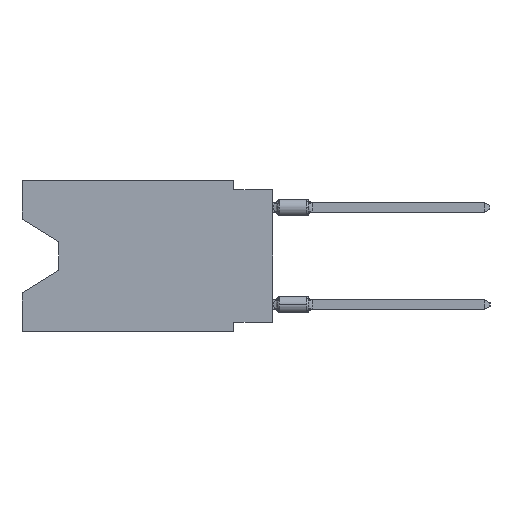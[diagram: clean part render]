
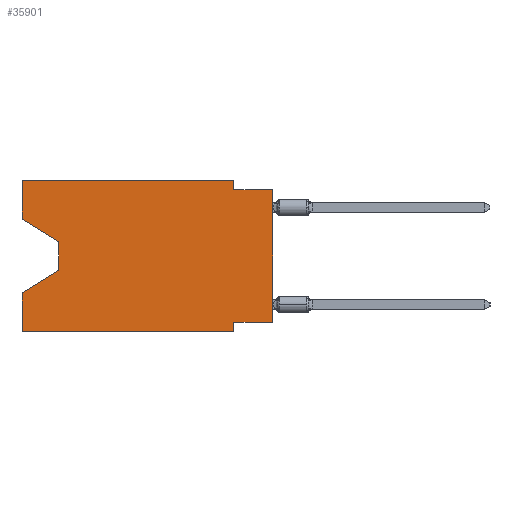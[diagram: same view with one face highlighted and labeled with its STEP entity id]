
A CAD part, left-side view. The second image highlights one B-rep face of the part: STEP entity #35901.
In plain terms, the highlighted planar face has unit normal (-1, 0, 0).
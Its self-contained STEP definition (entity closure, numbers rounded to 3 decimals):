
#434 = CARTESIAN_POINT ( 'NONE',  ( 0., 2.54, -9.271 ) ) ;
#891 = CARTESIAN_POINT ( 'NONE',  ( 0., 16.383, -9.906 ) ) ;
#1484 = LINE ( 'NONE', #5335, #4789 ) ;
#1598 = VECTOR ( 'NONE', #32664, 1000. ) ;
#1638 = CARTESIAN_POINT ( 'NONE',  ( 0., 2.54, -0.635 ) ) ;
#1687 = VERTEX_POINT ( 'NONE', #32587 ) ;
#2540 = VERTEX_POINT ( 'NONE', #35864 ) ;
#3015 = CARTESIAN_POINT ( 'NONE',  ( 0., 16.383, 0. ) ) ;
#3181 = DIRECTION ( 'NONE',  ( 0., -1., 0. ) ) ;
#3291 = DIRECTION ( 'NONE',  ( 0., 0., 1. ) ) ;
#3505 = CARTESIAN_POINT ( 'NONE',  ( 0., 16.383, 0. ) ) ;
#4196 = VERTEX_POINT ( 'NONE', #13522 ) ;
#4789 = VECTOR ( 'NONE', #21442, 1000. ) ;
#5096 = VECTOR ( 'NONE', #3291, 1000. ) ;
#5335 = CARTESIAN_POINT ( 'NONE',  ( 0., 0., 0. ) ) ;
#5982 = DIRECTION ( 'NONE',  ( 0., -1., 0. ) ) ;
#6082 = CARTESIAN_POINT ( 'NONE',  ( 0., 2.54, -9.906 ) ) ;
#6250 = LINE ( 'NONE', #3015, #32793 ) ;
#6885 = DIRECTION ( 'NONE',  ( 0., 0.855, -0.519 ) ) ;
#8403 = EDGE_CURVE ( 'NONE', #33445, #1687, #29652, .T. ) ;
#8707 = ORIENTED_EDGE ( 'NONE', *, *, #40645, .F. ) ;
#9124 = EDGE_CURVE ( 'NONE', #30574, #18743, #27374, .T. ) ;
#9193 = CARTESIAN_POINT ( 'NONE',  ( 0., 0., -0.635 ) ) ;
#9357 = EDGE_CURVE ( 'NONE', #30794, #33891, #23034, .T. ) ;
#9848 = CARTESIAN_POINT ( 'NONE',  ( 0., 0., -9.271 ) ) ;
#10131 = ORIENTED_EDGE ( 'NONE', *, *, #9357, .F. ) ;
#10392 = CARTESIAN_POINT ( 'NONE',  ( 0., 13.97, -4.013 ) ) ;
#10699 = AXIS2_PLACEMENT_3D ( 'NONE', #3505, #36114, #16602 ) ;
#10720 = VECTOR ( 'NONE', #6885, 1000. ) ;
#10819 = CARTESIAN_POINT ( 'NONE',  ( 0., 2.54, 0. ) ) ;
#11073 = CARTESIAN_POINT ( 'NONE',  ( 0., 16.383, 0. ) ) ;
#11210 = ORIENTED_EDGE ( 'NONE', *, *, #15955, .F. ) ;
#11588 = VERTEX_POINT ( 'NONE', #9848 ) ;
#12098 = LINE ( 'NONE', #35879, #12775 ) ;
#12408 = LINE ( 'NONE', #22470, #14924 ) ;
#12775 = VECTOR ( 'NONE', #42122, 1000. ) ;
#12973 = FACE_OUTER_BOUND ( 'NONE', #33775, .T. ) ;
#13182 = CARTESIAN_POINT ( 'NONE',  ( 0., 16.383, 0. ) ) ;
#13522 = CARTESIAN_POINT ( 'NONE',  ( 0., 0., -0.635 ) ) ;
#14281 = CARTESIAN_POINT ( 'NONE',  ( 0., 16.383, -2.546 ) ) ;
#14666 = VECTOR ( 'NONE', #3181, 1000. ) ;
#14673 = VECTOR ( 'NONE', #42078, 1000. ) ;
#14924 = VECTOR ( 'NONE', #35763, 1000. ) ;
#15955 = EDGE_CURVE ( 'NONE', #11588, #33445, #12408, .T. ) ;
#16110 = DIRECTION ( 'NONE',  ( 0., 0., 1. ) ) ;
#16602 = DIRECTION ( 'NONE',  ( 0., 0., -1. ) ) ;
#18743 = VERTEX_POINT ( 'NONE', #10819 ) ;
#19368 = VERTEX_POINT ( 'NONE', #22126 ) ;
#19757 = CARTESIAN_POINT ( 'NONE',  ( 0., 13.97, -5.893 ) ) ;
#20030 = VERTEX_POINT ( 'NONE', #1638 ) ;
#21188 = ORIENTED_EDGE ( 'NONE', *, *, #30206, .T. ) ;
#21442 = DIRECTION ( 'NONE',  ( 0., 0., 1. ) ) ;
#22126 = CARTESIAN_POINT ( 'NONE',  ( 0., 16.383, -2.546 ) ) ;
#22363 = VECTOR ( 'NONE', #5982, 1000. ) ;
#22470 = CARTESIAN_POINT ( 'NONE',  ( 0., 0., -9.271 ) ) ;
#23034 = LINE ( 'NONE', #13182, #5096 ) ;
#24138 = DIRECTION ( 'NONE',  ( 0., -0.855, -0.519 ) ) ;
#25065 = VECTOR ( 'NONE', #24138, 1000. ) ;
#25279 = VECTOR ( 'NONE', #32923, 1000. ) ;
#25491 = ORIENTED_EDGE ( 'NONE', *, *, #33327, .F. ) ;
#25559 = LINE ( 'NONE', #35420, #14673 ) ;
#25683 = EDGE_CURVE ( 'NONE', #30794, #1687, #12098, .T. ) ;
#26721 = EDGE_CURVE ( 'NONE', #19368, #2540, #33144, .T. ) ;
#27374 = LINE ( 'NONE', #11073, #14666 ) ;
#27464 = EDGE_CURVE ( 'NONE', #41547, #33891, #39259, .T. ) ;
#27594 = ORIENTED_EDGE ( 'NONE', *, *, #27464, .T. ) ;
#27815 = EDGE_CURVE ( 'NONE', #20030, #4196, #38573, .T. ) ;
#29008 = CARTESIAN_POINT ( 'NONE',  ( 0., 16.383, 0. ) ) ;
#29358 = CARTESIAN_POINT ( 'NONE',  ( 0., 16.383, -7.36 ) ) ;
#29652 = LINE ( 'NONE', #6082, #1598 ) ;
#30033 = ORIENTED_EDGE ( 'NONE', *, *, #8403, .F. ) ;
#30206 = EDGE_CURVE ( 'NONE', #2540, #41547, #39781, .T. ) ;
#30574 = VERTEX_POINT ( 'NONE', #29008 ) ;
#30794 = VERTEX_POINT ( 'NONE', #891 ) ;
#31306 = EDGE_CURVE ( 'NONE', #11588, #4196, #1484, .T. ) ;
#32587 = CARTESIAN_POINT ( 'NONE',  ( 0., 2.54, -9.906 ) ) ;
#32590 = ORIENTED_EDGE ( 'NONE', *, *, #9124, .F. ) ;
#32664 = DIRECTION ( 'NONE',  ( 0., 0., -1. ) ) ;
#32793 = VECTOR ( 'NONE', #16110, 1000. ) ;
#32923 = DIRECTION ( 'NONE',  ( 0., 0., -1. ) ) ;
#32932 = ORIENTED_EDGE ( 'NONE', *, *, #27815, .F. ) ;
#33144 = LINE ( 'NONE', #14281, #25065 ) ;
#33327 = EDGE_CURVE ( 'NONE', #18743, #20030, #25559, .T. ) ;
#33445 = VERTEX_POINT ( 'NONE', #434 ) ;
#33536 = CARTESIAN_POINT ( 'NONE',  ( 0., 13.97, -5.893 ) ) ;
#33775 = EDGE_LOOP ( 'NONE', ( #35401, #21188, #27594, #10131, #37641, #30033, #11210, #41013, #32932, #25491, #32590, #8707 ) ) ;
#33891 = VERTEX_POINT ( 'NONE', #29358 ) ;
#35401 = ORIENTED_EDGE ( 'NONE', *, *, #26721, .T. ) ;
#35420 = CARTESIAN_POINT ( 'NONE',  ( 0., 2.54, 0. ) ) ;
#35763 = DIRECTION ( 'NONE',  ( 0., 1., 0. ) ) ;
#35864 = CARTESIAN_POINT ( 'NONE',  ( 0., 13.97, -4.013 ) ) ;
#35879 = CARTESIAN_POINT ( 'NONE',  ( 0., 16.383, -9.906 ) ) ;
#35901 = ADVANCED_FACE ( 'NONE', ( #12973 ), #39326, .F. ) ;
#36114 = DIRECTION ( 'NONE',  ( 1., 0., 0. ) ) ;
#37641 = ORIENTED_EDGE ( 'NONE', *, *, #25683, .T. ) ;
#38573 = LINE ( 'NONE', #9193, #22363 ) ;
#39259 = LINE ( 'NONE', #19757, #10720 ) ;
#39326 = PLANE ( 'NONE',  #10699 ) ;
#39781 = LINE ( 'NONE', #10392, #25279 ) ;
#40645 = EDGE_CURVE ( 'NONE', #19368, #30574, #6250, .T. ) ;
#41013 = ORIENTED_EDGE ( 'NONE', *, *, #31306, .T. ) ;
#41547 = VERTEX_POINT ( 'NONE', #33536 ) ;
#42078 = DIRECTION ( 'NONE',  ( 0., 0., -1. ) ) ;
#42122 = DIRECTION ( 'NONE',  ( 0., -1., 0. ) ) ;
